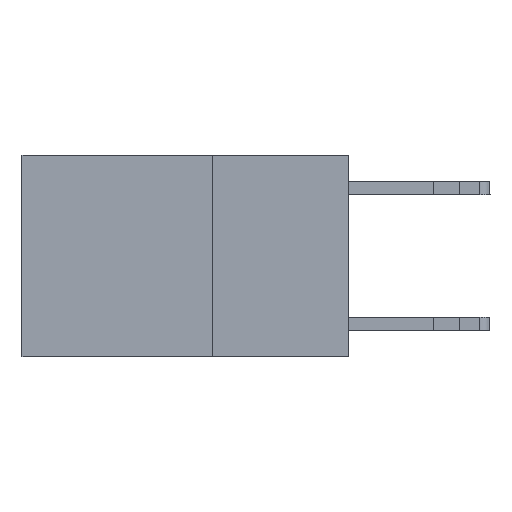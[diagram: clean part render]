
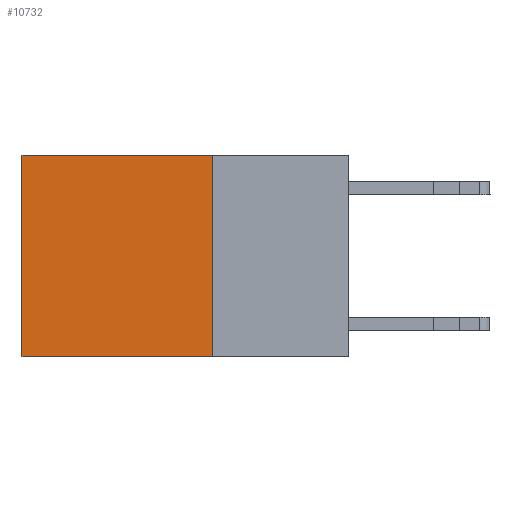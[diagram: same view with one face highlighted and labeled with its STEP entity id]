
A CAD part, left-side view. The second image highlights one B-rep face of the part: STEP entity #10732.
In plain terms, the highlighted planar face has unit normal (-1, 0, 0).
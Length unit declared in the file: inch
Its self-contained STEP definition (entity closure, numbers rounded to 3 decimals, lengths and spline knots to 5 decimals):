
#80 = VECTOR ( 'NONE', #10776, 39.37008 ) ;
#118 = VERTEX_POINT ( 'NONE', #6329 ) ;
#248 = ORIENTED_EDGE ( 'NONE', *, *, #5998, .F. ) ;
#687 = CARTESIAN_POINT ( 'NONE',  ( 0.2625, 0.25, 0. ) ) ;
#989 = ORIENTED_EDGE ( 'NONE', *, *, #4372, .T. ) ;
#1452 = ORIENTED_EDGE ( 'NONE', *, *, #6977, .T. ) ;
#1662 = DIRECTION ( 'NONE',  ( 0., 0., -1. ) ) ;
#2562 = VERTEX_POINT ( 'NONE', #10438 ) ;
#2978 = DIRECTION ( 'NONE',  ( 0., 1., 0. ) ) ;
#3103 = LINE ( 'NONE', #8309, #7836 ) ;
#3612 = FACE_OUTER_BOUND ( 'NONE', #9651, .T. ) ;
#4143 = CARTESIAN_POINT ( 'NONE',  ( 0.2625, 0.25, 0. ) ) ;
#4372 = EDGE_CURVE ( 'NONE', #2562, #7339, #10540, .T. ) ;
#5458 = LINE ( 'NONE', #4143, #80 ) ;
#5547 = CARTESIAN_POINT ( 'NONE',  ( 0.2625, 0.25, 0. ) ) ;
#5594 = ORIENTED_EDGE ( 'NONE', *, *, #5843, .F. ) ;
#5843 = EDGE_CURVE ( 'NONE', #118, #10820, #11411, .T. ) ;
#5923 = CARTESIAN_POINT ( 'NONE',  ( 0.2625, 0.6, 0. ) ) ;
#5998 = EDGE_CURVE ( 'NONE', #2562, #118, #5458, .T. ) ;
#6329 = CARTESIAN_POINT ( 'NONE',  ( 0.2625, 0.25, -0.37 ) ) ;
#6399 = PLANE ( 'NONE',  #11614 ) ;
#6977 = EDGE_CURVE ( 'NONE', #7339, #10820, #3103, .T. ) ;
#7339 = VERTEX_POINT ( 'NONE', #5923 ) ;
#7356 = DIRECTION ( 'NONE',  ( 1., 0., 0. ) ) ;
#7836 = VECTOR ( 'NONE', #9271, 39.37008 ) ;
#8024 = VECTOR ( 'NONE', #12198, 39.37008 ) ;
#8309 = CARTESIAN_POINT ( 'NONE',  ( 0.2625, 0.6, 0. ) ) ;
#8392 = CARTESIAN_POINT ( 'NONE',  ( 0.2625, 0.6, -0.37 ) ) ;
#8912 = VECTOR ( 'NONE', #2978, 39.37008 ) ;
#9271 = DIRECTION ( 'NONE',  ( 0., 0., -1. ) ) ;
#9651 = EDGE_LOOP ( 'NONE', ( #1452, #5594, #248, #989 ) ) ;
#10438 = CARTESIAN_POINT ( 'NONE',  ( 0.2625, 0.25, 0. ) ) ;
#10540 = LINE ( 'NONE', #5547, #8024 ) ;
#10732 = ADVANCED_FACE ( 'NONE', ( #3612 ), #6399, .F. ) ;
#10776 = DIRECTION ( 'NONE',  ( 0., 0., -1. ) ) ;
#10820 = VERTEX_POINT ( 'NONE', #8392 ) ;
#11411 = LINE ( 'NONE', #11465, #8912 ) ;
#11465 = CARTESIAN_POINT ( 'NONE',  ( 0.2625, 0.25, -0.37 ) ) ;
#11614 = AXIS2_PLACEMENT_3D ( 'NONE', #687, #7356, #1662 ) ;
#12198 = DIRECTION ( 'NONE',  ( 0., 1., 0. ) ) ;
